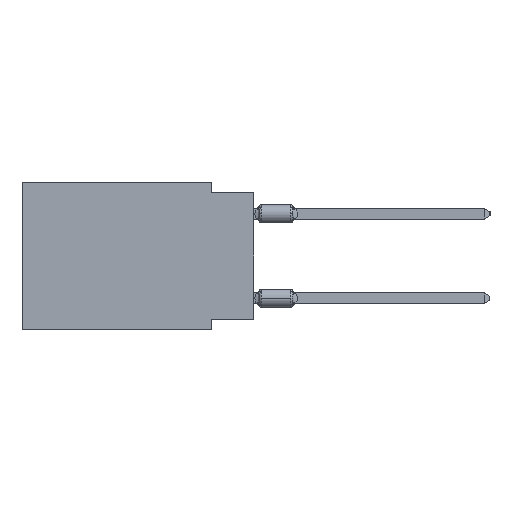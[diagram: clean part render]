
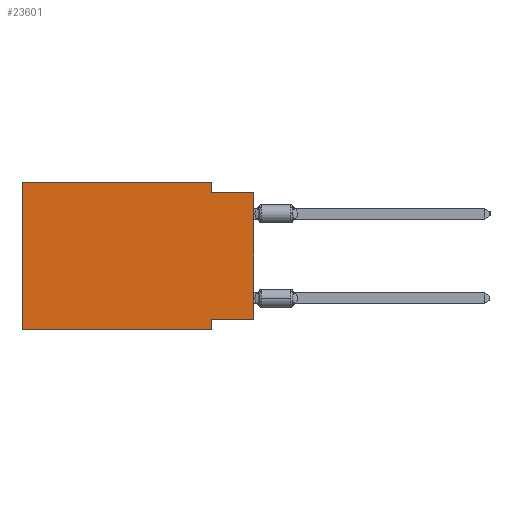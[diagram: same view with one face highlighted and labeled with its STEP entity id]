
A CAD part, left-side view. The second image highlights one B-rep face of the part: STEP entity #23601.
In plain terms, the highlighted planar face has unit normal (-1, 0, 0).
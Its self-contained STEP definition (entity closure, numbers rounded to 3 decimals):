
#281 = EDGE_CURVE ( 'NONE', #17454, #24499, #20224, .T. ) ;
#1038 = VECTOR ( 'NONE', #1739, 1000. ) ;
#1739 = DIRECTION ( 'NONE',  ( 0., 0., -1. ) ) ;
#5831 = CARTESIAN_POINT ( 'NONE',  ( 0., 13.97, 0. ) ) ;
#5930 = ORIENTED_EDGE ( 'NONE', *, *, #58934, .F. ) ;
#8248 = EDGE_CURVE ( 'NONE', #8949, #46168, #18047, .T. ) ;
#8645 = VECTOR ( 'NONE', #53291, 1000. ) ;
#8949 = VERTEX_POINT ( 'NONE', #65172 ) ;
#9000 = LINE ( 'NONE', #19305, #22713 ) ;
#10233 = DIRECTION ( 'NONE',  ( 0., -1., 0. ) ) ;
#13077 = EDGE_CURVE ( 'NONE', #13771, #26128, #9000, .T. ) ;
#13771 = VERTEX_POINT ( 'NONE', #29364 ) ;
#14589 = CARTESIAN_POINT ( 'NONE',  ( 0., 13.97, 0. ) ) ;
#15556 = DIRECTION ( 'NONE',  ( 0., 1., 0. ) ) ;
#17454 = VERTEX_POINT ( 'NONE', #40765 ) ;
#17729 = VECTOR ( 'NONE', #43056, 1000. ) ;
#18047 = LINE ( 'NONE', #28352, #8645 ) ;
#19305 = CARTESIAN_POINT ( 'NONE',  ( 0., 13.97, 0. ) ) ;
#20224 = LINE ( 'NONE', #40495, #37521 ) ;
#20543 = FACE_OUTER_BOUND ( 'NONE', #31908, .T. ) ;
#22445 = ORIENTED_EDGE ( 'NONE', *, *, #34274, .T. ) ;
#22713 = VECTOR ( 'NONE', #10233, 1000. ) ;
#23601 = ADVANCED_FACE ( 'NONE', ( #20543 ), #60134, .F. ) ;
#23893 = EDGE_CURVE ( 'NONE', #36908, #49877, #28136, .T. ) ;
#24066 = CARTESIAN_POINT ( 'NONE',  ( 0., 2.54, -8.255 ) ) ;
#24499 = VERTEX_POINT ( 'NONE', #24066 ) ;
#26128 = VERTEX_POINT ( 'NONE', #32896 ) ;
#28136 = LINE ( 'NONE', #44105, #39966 ) ;
#28352 = CARTESIAN_POINT ( 'NONE',  ( 0., 0., -0.635 ) ) ;
#29006 = EDGE_CURVE ( 'NONE', #24499, #49877, #65379, .T. ) ;
#29222 = CARTESIAN_POINT ( 'NONE',  ( 0., 2.54, -8.89 ) ) ;
#29364 = CARTESIAN_POINT ( 'NONE',  ( 0., 13.97, 0. ) ) ;
#31908 = EDGE_LOOP ( 'NONE', ( #22445, #39529, #65166, #57280, #5930, #40314, #42890, #36886 ) ) ;
#32896 = CARTESIAN_POINT ( 'NONE',  ( 0., 2.54, 0. ) ) ;
#33712 = DIRECTION ( 'NONE',  ( 0., 0., 1. ) ) ;
#34125 = CARTESIAN_POINT ( 'NONE',  ( 0., 2.54, -8.89 ) ) ;
#34274 = EDGE_CURVE ( 'NONE', #17454, #46168, #58344, .T. ) ;
#36886 = ORIENTED_EDGE ( 'NONE', *, *, #281, .F. ) ;
#36908 = VERTEX_POINT ( 'NONE', #63363 ) ;
#37521 = VECTOR ( 'NONE', #15556, 1000. ) ;
#38572 = VECTOR ( 'NONE', #33712, 1000. ) ;
#38760 = EDGE_CURVE ( 'NONE', #26128, #8949, #42288, .T. ) ;
#39529 = ORIENTED_EDGE ( 'NONE', *, *, #8248, .F. ) ;
#39966 = VECTOR ( 'NONE', #53742, 1000. ) ;
#40314 = ORIENTED_EDGE ( 'NONE', *, *, #23893, .T. ) ;
#40495 = CARTESIAN_POINT ( 'NONE',  ( 0., 0., -8.255 ) ) ;
#40765 = CARTESIAN_POINT ( 'NONE',  ( 0., 0., -8.255 ) ) ;
#42288 = LINE ( 'NONE', #62884, #1038 ) ;
#42890 = ORIENTED_EDGE ( 'NONE', *, *, #29006, .F. ) ;
#43056 = DIRECTION ( 'NONE',  ( 0., 0., 1. ) ) ;
#43706 = CARTESIAN_POINT ( 'NONE',  ( 0., 0., 0. ) ) ;
#44105 = CARTESIAN_POINT ( 'NONE',  ( 0., 13.97, -8.89 ) ) ;
#46168 = VERTEX_POINT ( 'NONE', #59373 ) ;
#49877 = VERTEX_POINT ( 'NONE', #29222 ) ;
#51364 = LINE ( 'NONE', #5831, #38572 ) ;
#53291 = DIRECTION ( 'NONE',  ( 0., -1., 0. ) ) ;
#53742 = DIRECTION ( 'NONE',  ( 0., -1., 0. ) ) ;
#56961 = AXIS2_PLACEMENT_3D ( 'NONE', #14589, #60766, #60458 ) ;
#57280 = ORIENTED_EDGE ( 'NONE', *, *, #13077, .F. ) ;
#58344 = LINE ( 'NONE', #43706, #17729 ) ;
#58934 = EDGE_CURVE ( 'NONE', #36908, #13771, #51364, .T. ) ;
#59373 = CARTESIAN_POINT ( 'NONE',  ( 0., 0., -0.635 ) ) ;
#60134 = PLANE ( 'NONE',  #56961 ) ;
#60458 = DIRECTION ( 'NONE',  ( 0., 0., -1. ) ) ;
#60766 = DIRECTION ( 'NONE',  ( 1., 0., 0. ) ) ;
#61538 = VECTOR ( 'NONE', #65053, 1000. ) ;
#62884 = CARTESIAN_POINT ( 'NONE',  ( 0., 2.54, 0. ) ) ;
#63363 = CARTESIAN_POINT ( 'NONE',  ( 0., 13.97, -8.89 ) ) ;
#65053 = DIRECTION ( 'NONE',  ( 0., 0., -1. ) ) ;
#65166 = ORIENTED_EDGE ( 'NONE', *, *, #38760, .F. ) ;
#65172 = CARTESIAN_POINT ( 'NONE',  ( 0., 2.54, -0.635 ) ) ;
#65379 = LINE ( 'NONE', #34125, #61538 ) ;
